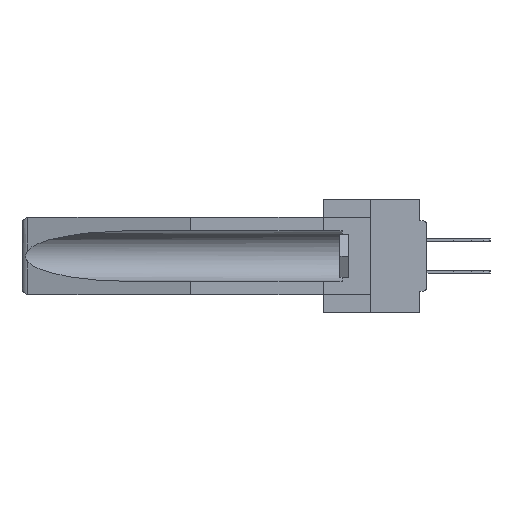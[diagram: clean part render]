
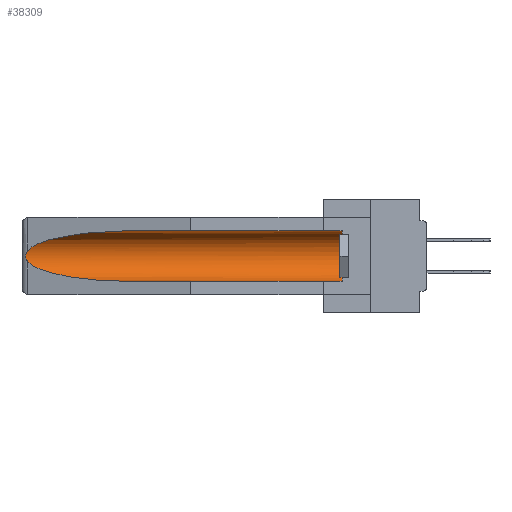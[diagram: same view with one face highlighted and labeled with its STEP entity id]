
A CAD part, left-side view. The second image highlights one B-rep face of the part: STEP entity #38309.
In plain terms, the highlighted cylindrical face has radius 2.857 mm (diameter 5.715 mm), a partial arc.
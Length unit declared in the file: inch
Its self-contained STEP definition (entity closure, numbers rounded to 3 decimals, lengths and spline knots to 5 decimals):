
#851 = CARTESIAN_POINT ( 'NONE',  ( 0.26597, 1.52961, -0.15275 ) ) ;
#1523 = CARTESIAN_POINT ( 'NONE',  ( 0.2673, 1.5327, -0.16383 ) ) ;
#2260 = VERTEX_POINT ( 'NONE', #31031 ) ;
#2662 = CARTESIAN_POINT ( 'NONE',  ( 0.155, -0.30754, -0.059 ) ) ;
#3027 = VERTEX_POINT ( 'NONE', #6548 ) ;
#3110 = CARTESIAN_POINT ( 'NONE',  ( 0.155, -0.30754, -0.284 ) ) ;
#3480 = FACE_OUTER_BOUND ( 'NONE', #19076, .T. ) ;
#5632 = LINE ( 'NONE', #2662, #34804 ) ;
#5857 = AXIS2_PLACEMENT_3D ( 'NONE', #7551, #35400, #16931 ) ;
#6548 = CARTESIAN_POINT ( 'NONE',  ( 0.155, 0.126, -0.059 ) ) ;
#6914 = EDGE_CURVE ( 'NONE', #25820, #13374, #31815, .T. ) ;
#7551 = CARTESIAN_POINT ( 'NONE',  ( 0.155, -0.30754, -0.1715 ) ) ;
#7780 = CARTESIAN_POINT ( 'NONE',  ( 0.2675, 1.53308, -0.16763 ) ) ;
#7912 = CARTESIAN_POINT ( 'NONE',  ( 0.2673, 1.53269, -0.17917 ) ) ;
#7920 = ORIENTED_EDGE ( 'NONE', *, *, #15098, .T. ) ;
#8496 = CARTESIAN_POINT ( 'NONE',  ( 0.26537, 1.52718, -0.14972 ) ) ;
#9497 = CARTESIAN_POINT ( 'NONE',  ( 0.25451, 1.48313, -0.24835 ) ) ;
#9670 = ORIENTED_EDGE ( 'NONE', *, *, #20529, .T. ) ;
#11726 = CARTESIAN_POINT ( 'NONE',  ( 0.155, 1.07973, -0.059 ) ) ;
#12124 = CARTESIAN_POINT ( 'NONE',  ( 0.155, 0.126, -0.284 ) ) ;
#12312 = ORIENTED_EDGE ( 'NONE', *, *, #17751, .F. ) ;
#12606 =( BOUNDED_CURVE ( )  B_SPLINE_CURVE ( 3, ( #11726, #20848, #24096, #8496 ),
 .UNSPECIFIED., .F., .F. ) 
 B_SPLINE_CURVE_WITH_KNOTS ( ( 4, 4 ),
 ( 4.71239, 6.08839 ),
 .UNSPECIFIED. ) 
 CURVE ( )  GEOMETRIC_REPRESENTATION_ITEM ( )  RATIONAL_B_SPLINE_CURVE ( ( 1., 0.848, 0.848, 1. ) ) 
 REPRESENTATION_ITEM ( '' )  );
#13291 = ORIENTED_EDGE ( 'NONE', *, *, #25061, .T. ) ;
#13374 = VERTEX_POINT ( 'NONE', #21023 ) ;
#13888 = CARTESIAN_POINT ( 'NONE',  ( 0.2675, 1.53308, -0.17534 ) ) ;
#14786 = DIRECTION ( 'NONE',  ( 0., -1., 0. ) ) ;
#14934 = CARTESIAN_POINT ( 'NONE',  ( 0.155, 0.126, -0.1715 ) ) ;
#15070 = DIRECTION ( 'NONE',  ( 0., 0., 1. ) ) ;
#15098 = EDGE_CURVE ( 'NONE', #3027, #32741, #5632, .T. ) ;
#16010 = CARTESIAN_POINT ( 'NONE',  ( 0.155, 1.07973, -0.284 ) ) ;
#16444 = ORIENTED_EDGE ( 'NONE', *, *, #22585, .T. ) ;
#16931 = DIRECTION ( 'NONE',  ( 0., 0., 1. ) ) ;
#17421 = CARTESIAN_POINT ( 'NONE',  ( 0.26597, 1.5296, -0.19026 ) ) ;
#17550 = CYLINDRICAL_SURFACE ( 'NONE', #5857, 0.1125 ) ;
#17751 = EDGE_CURVE ( 'NONE', #30756, #13374, #24892, .T. ) ;
#18095 = B_SPLINE_CURVE_WITH_KNOTS ( 'NONE', 3,
 ( #38465, #851, #20268, #1523, #7780, #13888, #7912, #35613, #17421, #20000 ),
 .UNSPECIFIED., .F., .F.,
 ( 4, 2, 2, 2, 4 ),
 ( 0., 0.00029, 0.00058, 0.00087, 0.00117 ),
 .UNSPECIFIED. ) ;
#18590 = DIRECTION ( 'NONE',  ( 0., 1., 0. ) ) ;
#18853 = ORIENTED_EDGE ( 'NONE', *, *, #6914, .T. ) ;
#18994 = CARTESIAN_POINT ( 'NONE',  ( 0.26537, 1.52718, -0.19328 ) ) ;
#19076 = EDGE_LOOP ( 'NONE', ( #13291, #16444, #18853, #12312, #9670, #7920 ) ) ;
#20000 = CARTESIAN_POINT ( 'NONE',  ( 0.26537, 1.52718, -0.19328 ) ) ;
#20268 = CARTESIAN_POINT ( 'NONE',  ( 0.26654, 1.53092, -0.15636 ) ) ;
#20529 = EDGE_CURVE ( 'NONE', #30756, #3027, #21929, .T. ) ;
#20848 = CARTESIAN_POINT ( 'NONE',  ( 0.21114, 1.30732, -0.059 ) ) ;
#21023 = CARTESIAN_POINT ( 'NONE',  ( 0.155, 1.07973, -0.284 ) ) ;
#21929 = CIRCLE ( 'NONE', #30218, 0.1125 ) ;
#22585 = EDGE_CURVE ( 'NONE', #2260, #25820, #18095, .T. ) ;
#24096 = CARTESIAN_POINT ( 'NONE',  ( 0.25451, 1.48313, -0.09465 ) ) ;
#24892 = LINE ( 'NONE', #3110, #35118 ) ;
#24980 = CARTESIAN_POINT ( 'NONE',  ( 0.26537, 1.52718, -0.19328 ) ) ;
#25061 = EDGE_CURVE ( 'NONE', #32741, #2260, #12606, .T. ) ;
#25820 = VERTEX_POINT ( 'NONE', #24980 ) ;
#30218 = AXIS2_PLACEMENT_3D ( 'NONE', #14934, #14786, #15070 ) ;
#30756 = VERTEX_POINT ( 'NONE', #12124 ) ;
#31031 = CARTESIAN_POINT ( 'NONE',  ( 0.26537, 1.52718, -0.14972 ) ) ;
#31815 =( BOUNDED_CURVE ( )  B_SPLINE_CURVE ( 3, ( #18994, #9497, #37868, #16010 ),
 .UNSPECIFIED., .F., .F. ) 
 B_SPLINE_CURVE_WITH_KNOTS ( ( 4, 4 ),
 ( 0.1948, 1.5708 ),
 .UNSPECIFIED. ) 
 CURVE ( )  GEOMETRIC_REPRESENTATION_ITEM ( )  RATIONAL_B_SPLINE_CURVE ( ( 1., 0.848, 0.848, 1. ) ) 
 REPRESENTATION_ITEM ( '' )  );
#32399 = CARTESIAN_POINT ( 'NONE',  ( 0.155, 1.07973, -0.059 ) ) ;
#32741 = VERTEX_POINT ( 'NONE', #32399 ) ;
#34804 = VECTOR ( 'NONE', #36475, 39.37008 ) ;
#35118 = VECTOR ( 'NONE', #18590, 39.37008 ) ;
#35400 = DIRECTION ( 'NONE',  ( 0., 1., 0. ) ) ;
#35613 = CARTESIAN_POINT ( 'NONE',  ( 0.26655, 1.53094, -0.18657 ) ) ;
#36475 = DIRECTION ( 'NONE',  ( 0., 1., 0. ) ) ;
#37868 = CARTESIAN_POINT ( 'NONE',  ( 0.21114, 1.30732, -0.284 ) ) ;
#38309 = ADVANCED_FACE ( 'NONE', ( #3480 ), #17550, .F. ) ;
#38465 = CARTESIAN_POINT ( 'NONE',  ( 0.26537, 1.52718, -0.14972 ) ) ;
